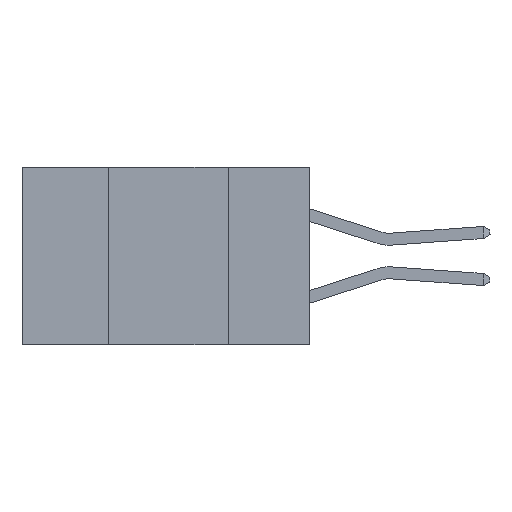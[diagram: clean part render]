
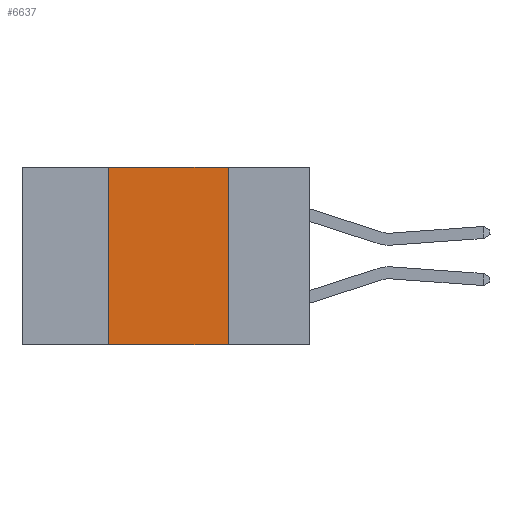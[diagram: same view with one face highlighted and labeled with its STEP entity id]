
A CAD part, left-side view. The second image highlights one B-rep face of the part: STEP entity #6637.
In plain terms, the highlighted planar face has unit normal (-1, 0, 0).
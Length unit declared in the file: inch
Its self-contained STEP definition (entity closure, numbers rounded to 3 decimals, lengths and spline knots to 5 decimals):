
#293 = LINE ( 'NONE', #5517, #20887 ) ;
#915 = EDGE_LOOP ( 'NONE', ( #17666, #1645, #16462, #6082 ) ) ;
#1622 = EDGE_CURVE ( 'NONE', #16389, #24163, #14335, .T. ) ;
#1645 = ORIENTED_EDGE ( 'NONE', *, *, #5803, .F. ) ;
#1863 = LINE ( 'NONE', #5745, #22350 ) ;
#2433 = EDGE_CURVE ( 'NONE', #25577, #24163, #16159, .T. ) ;
#2799 = DIRECTION ( 'NONE',  ( 0., -1., 0. ) ) ;
#3759 = VECTOR ( 'NONE', #23713, 39.37008 ) ;
#3817 = DIRECTION ( 'NONE',  ( 0., -1., 0. ) ) ;
#4967 = VECTOR ( 'NONE', #2799, 39.37008 ) ;
#5517 = CARTESIAN_POINT ( 'NONE',  ( 0., 0.6, 0. ) ) ;
#5745 = CARTESIAN_POINT ( 'NONE',  ( 0., 0.42, 0. ) ) ;
#5803 = EDGE_CURVE ( 'NONE', #17724, #16389, #293, .T. ) ;
#6082 = ORIENTED_EDGE ( 'NONE', *, *, #2433, .T. ) ;
#6320 = CARTESIAN_POINT ( 'NONE',  ( 0., 0.42, 0. ) ) ;
#6637 = ADVANCED_FACE ( 'NONE', ( #17206 ), #15342, .F. ) ;
#7476 = EDGE_CURVE ( 'NONE', #25577, #17724, #1863, .T. ) ;
#8987 = AXIS2_PLACEMENT_3D ( 'NONE', #9891, #19975, #18127 ) ;
#9891 = CARTESIAN_POINT ( 'NONE',  ( 0., 0.6, 0. ) ) ;
#10204 = CARTESIAN_POINT ( 'NONE',  ( 0., 0.17, -0.37 ) ) ;
#11569 = CARTESIAN_POINT ( 'NONE',  ( 0., 0.42, -0.37 ) ) ;
#14335 = LINE ( 'NONE', #25067, #3759 ) ;
#15342 = PLANE ( 'NONE',  #8987 ) ;
#15935 = CARTESIAN_POINT ( 'NONE',  ( 0., 0.17, 0. ) ) ;
#16159 = LINE ( 'NONE', #18859, #4967 ) ;
#16389 = VERTEX_POINT ( 'NONE', #15935 ) ;
#16462 = ORIENTED_EDGE ( 'NONE', *, *, #7476, .F. ) ;
#17206 = FACE_OUTER_BOUND ( 'NONE', #915, .T. ) ;
#17666 = ORIENTED_EDGE ( 'NONE', *, *, #1622, .F. ) ;
#17724 = VERTEX_POINT ( 'NONE', #6320 ) ;
#18127 = DIRECTION ( 'NONE',  ( 0., 0., -1. ) ) ;
#18859 = CARTESIAN_POINT ( 'NONE',  ( 0., 0.6, -0.37 ) ) ;
#19975 = DIRECTION ( 'NONE',  ( 1., 0., 0. ) ) ;
#20887 = VECTOR ( 'NONE', #3817, 39.37008 ) ;
#22350 = VECTOR ( 'NONE', #23485, 39.37008 ) ;
#23485 = DIRECTION ( 'NONE',  ( 0., 0., 1. ) ) ;
#23713 = DIRECTION ( 'NONE',  ( 0., 0., -1. ) ) ;
#24163 = VERTEX_POINT ( 'NONE', #10204 ) ;
#25067 = CARTESIAN_POINT ( 'NONE',  ( 0., 0.17, 0. ) ) ;
#25577 = VERTEX_POINT ( 'NONE', #11569 ) ;
